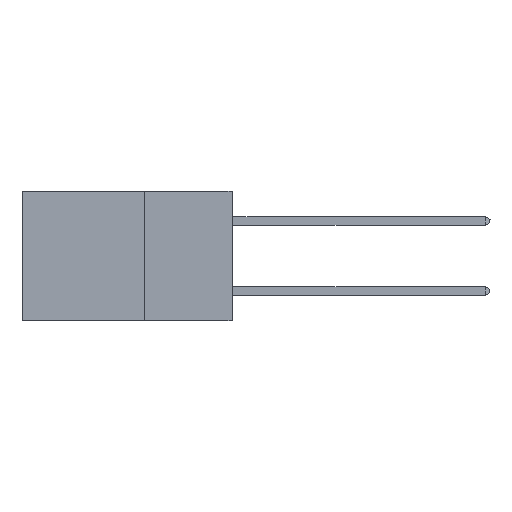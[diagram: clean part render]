
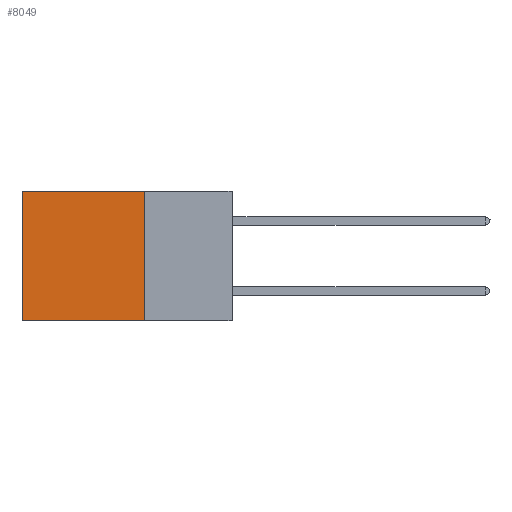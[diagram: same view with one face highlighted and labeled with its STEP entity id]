
A CAD part, left-side view. The second image highlights one B-rep face of the part: STEP entity #8049.
In plain terms, the highlighted planar face has unit normal (-1, 0, 0).
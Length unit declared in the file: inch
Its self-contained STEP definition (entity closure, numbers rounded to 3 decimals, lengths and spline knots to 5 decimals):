
#139 = LINE ( 'NONE', #1507, #12236 ) ;
#729 = CARTESIAN_POINT ( 'NONE',  ( 0.2875, 0.6, 0. ) ) ;
#812 = CARTESIAN_POINT ( 'NONE',  ( 0.2875, 0.6, -0.37 ) ) ;
#1055 = EDGE_CURVE ( 'NONE', #7233, #4857, #9303, .T. ) ;
#1507 = CARTESIAN_POINT ( 'NONE',  ( 0.2875, 0.25, 0. ) ) ;
#1928 = VECTOR ( 'NONE', #15806, 39.37008 ) ;
#1993 = LINE ( 'NONE', #8715, #8081 ) ;
#2377 = ORIENTED_EDGE ( 'NONE', *, *, #16571, .T. ) ;
#2441 = CARTESIAN_POINT ( 'NONE',  ( 0.2875, 0.6, 0. ) ) ;
#4850 = DIRECTION ( 'NONE',  ( 0., 0., -1. ) ) ;
#4857 = VERTEX_POINT ( 'NONE', #16369 ) ;
#5326 = AXIS2_PLACEMENT_3D ( 'NONE', #15673, #9002, #12927 ) ;
#5678 = CARTESIAN_POINT ( 'NONE',  ( 0.2875, 0.25, 0. ) ) ;
#6736 = PLANE ( 'NONE',  #5326 ) ;
#7233 = VERTEX_POINT ( 'NONE', #5678 ) ;
#7820 = ORIENTED_EDGE ( 'NONE', *, *, #13501, .F. ) ;
#7962 = FACE_OUTER_BOUND ( 'NONE', #13923, .T. ) ;
#8049 = ADVANCED_FACE ( 'NONE', ( #7962 ), #6736, .F. ) ;
#8081 = VECTOR ( 'NONE', #9923, 39.37008 ) ;
#8332 = VERTEX_POINT ( 'NONE', #729 ) ;
#8715 = CARTESIAN_POINT ( 'NONE',  ( 0.2875, 0.25, -0.37 ) ) ;
#8819 = LINE ( 'NONE', #2441, #8987 ) ;
#8987 = VECTOR ( 'NONE', #4850, 39.37008 ) ;
#9002 = DIRECTION ( 'NONE',  ( 1., 0., 0. ) ) ;
#9303 = LINE ( 'NONE', #14509, #1928 ) ;
#9923 = DIRECTION ( 'NONE',  ( 0., 1., 0. ) ) ;
#10685 = ORIENTED_EDGE ( 'NONE', *, *, #14987, .T. ) ;
#12236 = VECTOR ( 'NONE', #15846, 39.37008 ) ;
#12927 = DIRECTION ( 'NONE',  ( 0., 0., -1. ) ) ;
#13501 = EDGE_CURVE ( 'NONE', #4857, #16562, #1993, .T. ) ;
#13642 = ORIENTED_EDGE ( 'NONE', *, *, #1055, .F. ) ;
#13923 = EDGE_LOOP ( 'NONE', ( #2377, #7820, #13642, #10685 ) ) ;
#14509 = CARTESIAN_POINT ( 'NONE',  ( 0.2875, 0.25, 0. ) ) ;
#14987 = EDGE_CURVE ( 'NONE', #7233, #8332, #139, .T. ) ;
#15673 = CARTESIAN_POINT ( 'NONE',  ( 0.2875, 0.25, 0. ) ) ;
#15806 = DIRECTION ( 'NONE',  ( 0., 0., -1. ) ) ;
#15846 = DIRECTION ( 'NONE',  ( 0., 1., 0. ) ) ;
#16369 = CARTESIAN_POINT ( 'NONE',  ( 0.2875, 0.25, -0.37 ) ) ;
#16562 = VERTEX_POINT ( 'NONE', #812 ) ;
#16571 = EDGE_CURVE ( 'NONE', #8332, #16562, #8819, .T. ) ;
